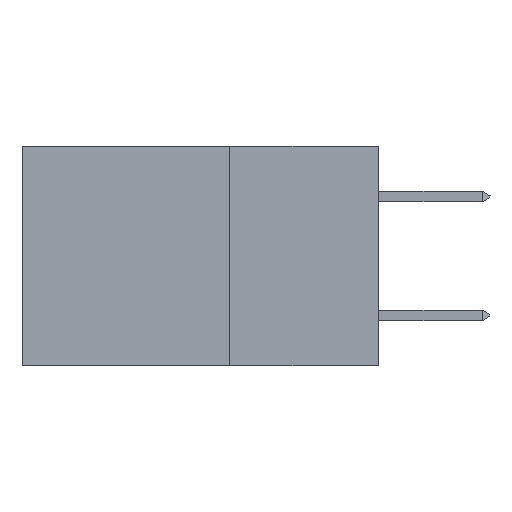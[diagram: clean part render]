
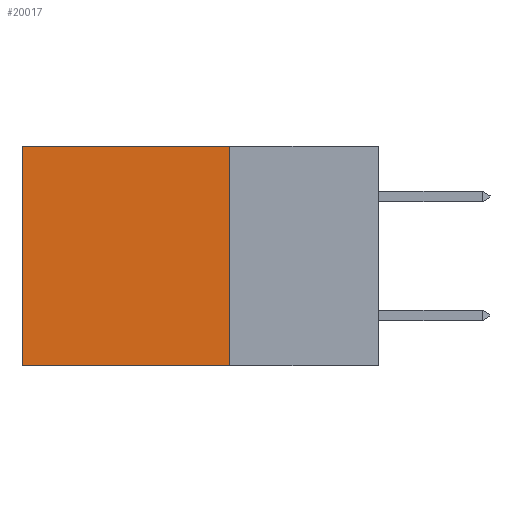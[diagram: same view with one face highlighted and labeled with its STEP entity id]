
A CAD part, left-side view. The second image highlights one B-rep face of the part: STEP entity #20017.
In plain terms, the highlighted planar face has unit normal (-1, 0, 0).
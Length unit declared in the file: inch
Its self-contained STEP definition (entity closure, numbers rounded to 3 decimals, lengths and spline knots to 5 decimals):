
#166 = DIRECTION ( 'NONE',  ( 0., 0., -1. ) ) ;
#290 = CARTESIAN_POINT ( 'NONE',  ( 0.2615, 0.25, 0. ) ) ;
#374 = DIRECTION ( 'NONE',  ( 0., 0., -1. ) ) ;
#971 = ORIENTED_EDGE ( 'NONE', *, *, #4267, .F. ) ;
#1751 = CARTESIAN_POINT ( 'NONE',  ( 0.2615, 0.25, -0.37 ) ) ;
#1890 = CARTESIAN_POINT ( 'NONE',  ( 0.2615, 0.25, -0.37 ) ) ;
#2187 = LINE ( 'NONE', #11529, #13036 ) ;
#3166 = VECTOR ( 'NONE', #14551, 39.37008 ) ;
#3825 = CARTESIAN_POINT ( 'NONE',  ( 0.2615, 0.25, 0. ) ) ;
#4009 = LINE ( 'NONE', #20091, #12011 ) ;
#4230 = EDGE_CURVE ( 'NONE', #10361, #5354, #9953, .T. ) ;
#4267 = EDGE_CURVE ( 'NONE', #10361, #9807, #19334, .T. ) ;
#5295 = EDGE_CURVE ( 'NONE', #9807, #5902, #4009, .T. ) ;
#5354 = VERTEX_POINT ( 'NONE', #7735 ) ;
#5902 = VERTEX_POINT ( 'NONE', #19269 ) ;
#7735 = CARTESIAN_POINT ( 'NONE',  ( 0.2615, 0.6, 0. ) ) ;
#8364 = DIRECTION ( 'NONE',  ( 0., 0., -1. ) ) ;
#9187 = CARTESIAN_POINT ( 'NONE',  ( 0.2615, 0.25, -0.37 ) ) ;
#9600 = EDGE_CURVE ( 'NONE', #5354, #5902, #2187, .T. ) ;
#9807 = VERTEX_POINT ( 'NONE', #9187 ) ;
#9821 = FACE_OUTER_BOUND ( 'NONE', #11527, .T. ) ;
#9847 = ORIENTED_EDGE ( 'NONE', *, *, #5295, .F. ) ;
#9953 = LINE ( 'NONE', #290, #3166 ) ;
#10361 = VERTEX_POINT ( 'NONE', #3825 ) ;
#11527 = EDGE_LOOP ( 'NONE', ( #19650, #9847, #971, #13378 ) ) ;
#11529 = CARTESIAN_POINT ( 'NONE',  ( 0.2615, 0.6, -0.37 ) ) ;
#11994 = DIRECTION ( 'NONE',  ( 0., 1., 0. ) ) ;
#12011 = VECTOR ( 'NONE', #11994, 39.37008 ) ;
#13036 = VECTOR ( 'NONE', #374, 39.37008 ) ;
#13378 = ORIENTED_EDGE ( 'NONE', *, *, #4230, .T. ) ;
#14031 = VECTOR ( 'NONE', #8364, 39.37008 ) ;
#14551 = DIRECTION ( 'NONE',  ( 0., 1., 0. ) ) ;
#14727 = DIRECTION ( 'NONE',  ( 1., 0., 0. ) ) ;
#15408 = AXIS2_PLACEMENT_3D ( 'NONE', #1751, #14727, #166 ) ;
#16329 = PLANE ( 'NONE',  #15408 ) ;
#19269 = CARTESIAN_POINT ( 'NONE',  ( 0.2615, 0.6, -0.37 ) ) ;
#19334 = LINE ( 'NONE', #1890, #14031 ) ;
#19650 = ORIENTED_EDGE ( 'NONE', *, *, #9600, .T. ) ;
#20017 = ADVANCED_FACE ( 'NONE', ( #9821 ), #16329, .F. ) ;
#20091 = CARTESIAN_POINT ( 'NONE',  ( 0.2615, 0.25, -0.37 ) ) ;
